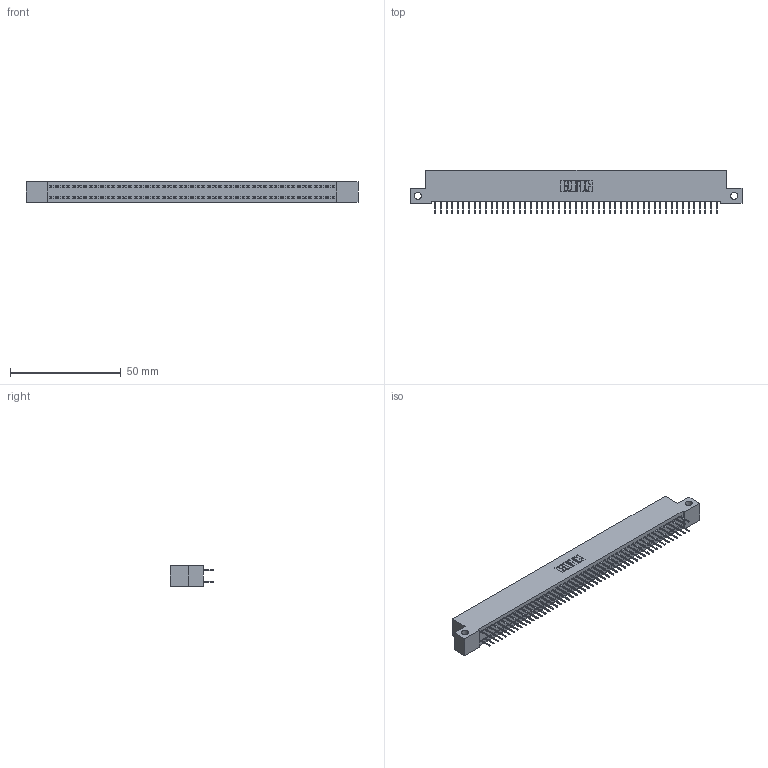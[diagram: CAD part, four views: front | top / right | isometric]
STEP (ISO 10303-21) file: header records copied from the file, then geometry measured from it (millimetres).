
FILE_DESCRIPTION (( 'STEP AP203' ), '1' );
FILE_NAME ('392-102-524-212.STEP', '2019-10-09T21:22:06', ( '' ), ( '' ), 'SwSTEP 2.0', 'SolidWorks 2016', '' );
FILE_SCHEMA (( 'CONFIG_CONTROL_DESIGN' ));
Length unit declared in the file: inch
Products named in the file (3): 342 Part_Side Mount; 345-292-001_345-293-124; 392-102-524-212
Assembly tree (103 placements, depth 2):
  392-102-524-212
    342 Part_Side Mount
    345-292-001_345-293-124  x102
Bounding box: 149.86 x 19.69 x 9.4 mm (x, y, z)
Volume: 13279.2 mm3; surface area: 21275.7 mm2
Topology: 103 solids, 103 shells, 5822 faces, 16517 edges, 10602 vertices
Faces by surface type: plane 4350, cylinder 1472
Entity records: 31591 total; most frequent: CARTESIAN_POINT 5222, ORIENTED_EDGE 5158, DIRECTION 4447, EDGE_CURVE 2579, LINE 2455, VECTOR 2455, VERTEX_POINT 1714, AXIS2_PLACEMENT_3D 996
